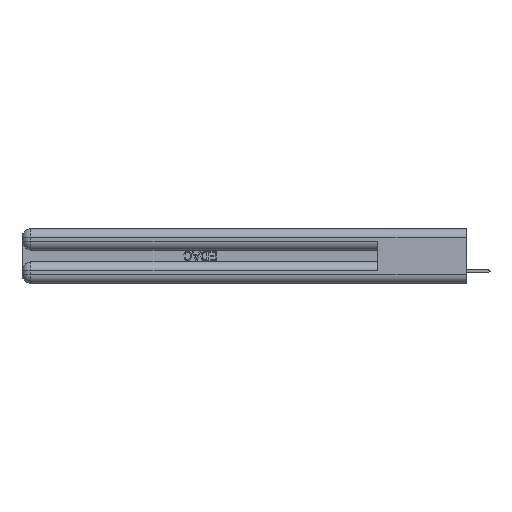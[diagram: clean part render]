
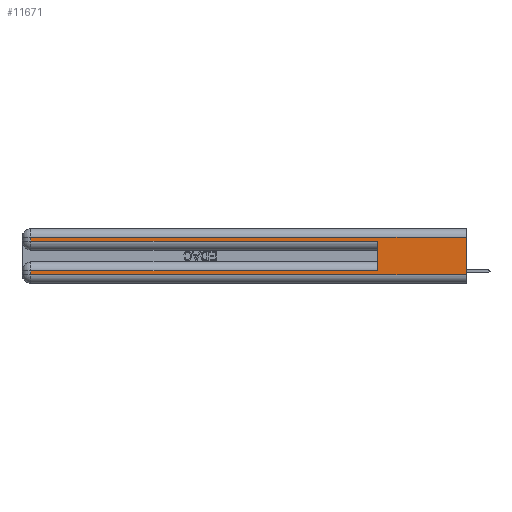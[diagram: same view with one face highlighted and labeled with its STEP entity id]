
A CAD part, left-side view. The second image highlights one B-rep face of the part: STEP entity #11671.
In plain terms, the highlighted planar face has unit normal (-1, 0, 0).
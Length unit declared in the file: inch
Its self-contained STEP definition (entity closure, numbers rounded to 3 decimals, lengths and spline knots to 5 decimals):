
#1018 = CARTESIAN_POINT ( 'NONE',  ( 0., 0.6, 0.085 ) ) ;
#1129 = DIRECTION ( 'NONE',  ( 0., 1., 0. ) ) ;
#1287 = CARTESIAN_POINT ( 'NONE',  ( 0., 0., 0.31 ) ) ;
#1925 = VERTEX_POINT ( 'NONE', #20792 ) ;
#2146 = VECTOR ( 'NONE', #19899, 39.37008 ) ;
#2588 = VERTEX_POINT ( 'NONE', #8570 ) ;
#3297 = LINE ( 'NONE', #36609, #30394 ) ;
#3374 = ORIENTED_EDGE ( 'NONE', *, *, #18053, .F. ) ;
#4486 = DIRECTION ( 'NONE',  ( 0., -1., 0. ) ) ;
#5500 = DIRECTION ( 'NONE',  ( 0., -1., 0. ) ) ;
#5655 = ORIENTED_EDGE ( 'NONE', *, *, #9777, .T. ) ;
#6023 = ORIENTED_EDGE ( 'NONE', *, *, #10716, .T. ) ;
#6541 = LINE ( 'NONE', #9347, #40304 ) ;
#6984 = VERTEX_POINT ( 'NONE', #1018 ) ;
#7218 = LINE ( 'NONE', #29719, #2146 ) ;
#7634 = LINE ( 'NONE', #1287, #10713 ) ;
#8118 = VECTOR ( 'NONE', #11820, 39.37008 ) ;
#8570 = CARTESIAN_POINT ( 'NONE',  ( 0., 2.94, 0.06 ) ) ;
#9329 = LINE ( 'NONE', #38936, #25688 ) ;
#9347 = CARTESIAN_POINT ( 'NONE',  ( 0., 0., 0.37 ) ) ;
#9777 = EDGE_CURVE ( 'NONE', #12229, #1925, #22815, .T. ) ;
#10713 = VECTOR ( 'NONE', #21550, 39.37008 ) ;
#10716 = EDGE_CURVE ( 'NONE', #2588, #37904, #39153, .T. ) ;
#11671 = ADVANCED_FACE ( 'NONE', ( #32218 ), #31906, .F. ) ;
#11734 = CARTESIAN_POINT ( 'NONE',  ( 0., 2.94, 0.31 ) ) ;
#11820 = DIRECTION ( 'NONE',  ( 0., 0., -1. ) ) ;
#12229 = VERTEX_POINT ( 'NONE', #28818 ) ;
#12958 = AXIS2_PLACEMENT_3D ( 'NONE', #13659, #30734, #20557 ) ;
#13294 = ORIENTED_EDGE ( 'NONE', *, *, #29697, .T. ) ;
#13659 = CARTESIAN_POINT ( 'NONE',  ( 0., 0., 0.37 ) ) ;
#14104 = CARTESIAN_POINT ( 'NONE',  ( 0., 0., 0.285 ) ) ;
#15304 = ORIENTED_EDGE ( 'NONE', *, *, #36895, .F. ) ;
#16947 = VERTEX_POINT ( 'NONE', #11734 ) ;
#18053 = EDGE_CURVE ( 'NONE', #18563, #37904, #6541, .T. ) ;
#18563 = VERTEX_POINT ( 'NONE', #30410 ) ;
#19899 = DIRECTION ( 'NONE',  ( 0., 0., -1. ) ) ;
#20557 = DIRECTION ( 'NONE',  ( 0., 0., -1. ) ) ;
#20792 = CARTESIAN_POINT ( 'NONE',  ( 0., 0.6, 0.285 ) ) ;
#21329 = VECTOR ( 'NONE', #4486, 39.37008 ) ;
#21547 = CARTESIAN_POINT ( 'NONE',  ( 0., 2.94, 0.37 ) ) ;
#21550 = DIRECTION ( 'NONE',  ( 0., 1., 0. ) ) ;
#22499 = DIRECTION ( 'NONE',  ( 0., 0., 1. ) ) ;
#22815 = LINE ( 'NONE', #14104, #21329 ) ;
#23880 = EDGE_CURVE ( 'NONE', #16947, #12229, #35735, .T. ) ;
#24534 = CARTESIAN_POINT ( 'NONE',  ( 0., 0., 0.06 ) ) ;
#25118 = DIRECTION ( 'NONE',  ( 0., 0., -1. ) ) ;
#25688 = VECTOR ( 'NONE', #22499, 39.37008 ) ;
#26779 = CARTESIAN_POINT ( 'NONE',  ( 0., 2.94, 0.085 ) ) ;
#26803 = VECTOR ( 'NONE', #5500, 39.37008 ) ;
#28818 = CARTESIAN_POINT ( 'NONE',  ( 0., 2.94, 0.285 ) ) ;
#29006 = VERTEX_POINT ( 'NONE', #26779 ) ;
#29083 = ORIENTED_EDGE ( 'NONE', *, *, #37811, .T. ) ;
#29697 = EDGE_CURVE ( 'NONE', #6984, #29006, #3297, .T. ) ;
#29719 = CARTESIAN_POINT ( 'NONE',  ( 0., 2.94, 0.37 ) ) ;
#30394 = VECTOR ( 'NONE', #1129, 39.37008 ) ;
#30410 = CARTESIAN_POINT ( 'NONE',  ( 0., 0., 0.31 ) ) ;
#30734 = DIRECTION ( 'NONE',  ( 1., 0., 0. ) ) ;
#31906 = PLANE ( 'NONE',  #12958 ) ;
#32218 = FACE_OUTER_BOUND ( 'NONE', #34173, .T. ) ;
#33178 = EDGE_CURVE ( 'NONE', #29006, #2588, #7218, .T. ) ;
#34173 = EDGE_LOOP ( 'NONE', ( #3374, #29083, #38034, #5655, #15304, #13294, #41560, #6023 ) ) ;
#34651 = CARTESIAN_POINT ( 'NONE',  ( 0., 0., 0.06 ) ) ;
#35735 = LINE ( 'NONE', #21547, #8118 ) ;
#36609 = CARTESIAN_POINT ( 'NONE',  ( 0., 0., 0.085 ) ) ;
#36895 = EDGE_CURVE ( 'NONE', #6984, #1925, #9329, .T. ) ;
#37811 = EDGE_CURVE ( 'NONE', #18563, #16947, #7634, .T. ) ;
#37904 = VERTEX_POINT ( 'NONE', #34651 ) ;
#38034 = ORIENTED_EDGE ( 'NONE', *, *, #23880, .T. ) ;
#38936 = CARTESIAN_POINT ( 'NONE',  ( 0., 0.6, 0.145 ) ) ;
#39153 = LINE ( 'NONE', #24534, #26803 ) ;
#40304 = VECTOR ( 'NONE', #25118, 39.37008 ) ;
#41560 = ORIENTED_EDGE ( 'NONE', *, *, #33178, .T. ) ;
